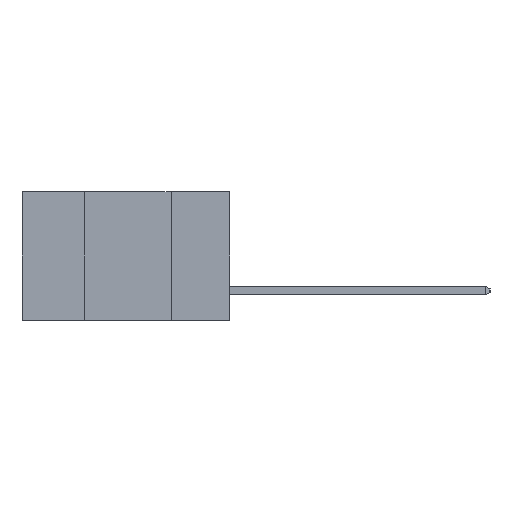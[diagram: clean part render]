
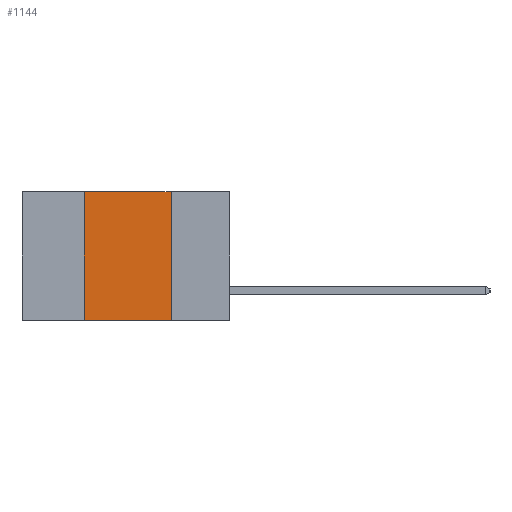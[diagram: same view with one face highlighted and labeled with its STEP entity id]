
A CAD part, left-side view. The second image highlights one B-rep face of the part: STEP entity #1144.
In plain terms, the highlighted planar face has unit normal (-1, 0, 0).
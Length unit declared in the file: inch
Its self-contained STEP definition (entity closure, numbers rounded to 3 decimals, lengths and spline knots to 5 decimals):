
#186 = VERTEX_POINT ( 'NONE', #7183 ) ;
#749 = VECTOR ( 'NONE', #6681, 39.37008 ) ;
#1144 = ADVANCED_FACE ( 'NONE', ( #8998 ), #1763, .F. ) ;
#1220 = VECTOR ( 'NONE', #6164, 39.37008 ) ;
#1461 = EDGE_CURVE ( 'NONE', #186, #10698, #9770, .T. ) ;
#1763 = PLANE ( 'NONE',  #10845 ) ;
#2429 = VERTEX_POINT ( 'NONE', #3914 ) ;
#2514 = CARTESIAN_POINT ( 'NONE',  ( 0., 0.17, -0.37 ) ) ;
#2681 = EDGE_CURVE ( 'NONE', #186, #2429, #5022, .T. ) ;
#2879 = VECTOR ( 'NONE', #8441, 39.37008 ) ;
#3239 = EDGE_CURVE ( 'NONE', #2429, #4293, #5403, .T. ) ;
#3390 = DIRECTION ( 'NONE',  ( 0., 0., 1. ) ) ;
#3669 = ORIENTED_EDGE ( 'NONE', *, *, #1461, .T. ) ;
#3811 = EDGE_CURVE ( 'NONE', #4293, #10698, #11004, .T. ) ;
#3914 = CARTESIAN_POINT ( 'NONE',  ( 0., 0.42, 0. ) ) ;
#4039 = CARTESIAN_POINT ( 'NONE',  ( 0., 0.17, 0. ) ) ;
#4293 = VERTEX_POINT ( 'NONE', #4039 ) ;
#5022 = LINE ( 'NONE', #9301, #9234 ) ;
#5391 = ORIENTED_EDGE ( 'NONE', *, *, #3239, .F. ) ;
#5403 = LINE ( 'NONE', #7535, #749 ) ;
#5824 = DIRECTION ( 'NONE',  ( 1., 0., 0. ) ) ;
#6164 = DIRECTION ( 'NONE',  ( 0., -1., 0. ) ) ;
#6299 = CARTESIAN_POINT ( 'NONE',  ( 0., 0.6, 0. ) ) ;
#6371 = EDGE_LOOP ( 'NONE', ( #7892, #5391, #8884, #3669 ) ) ;
#6681 = DIRECTION ( 'NONE',  ( 0., -1., 0. ) ) ;
#6789 = DIRECTION ( 'NONE',  ( 0., 0., -1. ) ) ;
#7183 = CARTESIAN_POINT ( 'NONE',  ( 0., 0.42, -0.37 ) ) ;
#7535 = CARTESIAN_POINT ( 'NONE',  ( 0., 0.6, 0. ) ) ;
#7892 = ORIENTED_EDGE ( 'NONE', *, *, #3811, .F. ) ;
#8218 = CARTESIAN_POINT ( 'NONE',  ( 0., 0.17, -0.37 ) ) ;
#8441 = DIRECTION ( 'NONE',  ( 0., 0., -1. ) ) ;
#8884 = ORIENTED_EDGE ( 'NONE', *, *, #2681, .F. ) ;
#8998 = FACE_OUTER_BOUND ( 'NONE', #6371, .T. ) ;
#9234 = VECTOR ( 'NONE', #3390, 39.37008 ) ;
#9301 = CARTESIAN_POINT ( 'NONE',  ( 0., 0.42, -0.37 ) ) ;
#9770 = LINE ( 'NONE', #10325, #1220 ) ;
#10325 = CARTESIAN_POINT ( 'NONE',  ( 0., 0.6, -0.37 ) ) ;
#10698 = VERTEX_POINT ( 'NONE', #8218 ) ;
#10845 = AXIS2_PLACEMENT_3D ( 'NONE', #6299, #5824, #6789 ) ;
#11004 = LINE ( 'NONE', #2514, #2879 ) ;
